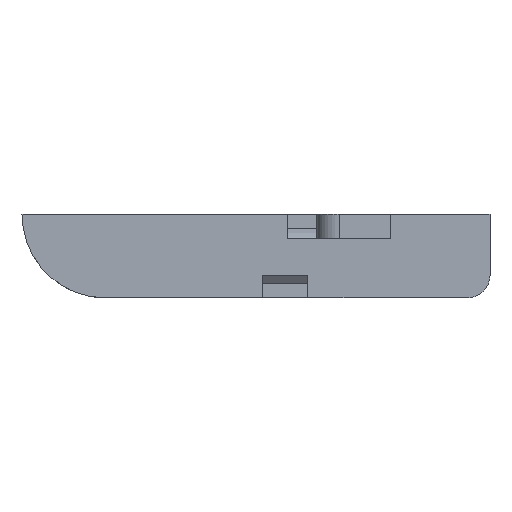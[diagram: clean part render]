
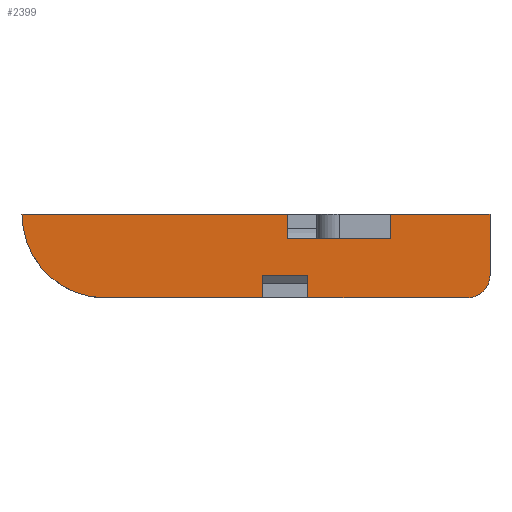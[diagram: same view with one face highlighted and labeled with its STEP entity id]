
A CAD part, left-side view. The second image highlights one B-rep face of the part: STEP entity #2399.
In plain terms, the highlighted planar face has unit normal (-1, 0, 0).
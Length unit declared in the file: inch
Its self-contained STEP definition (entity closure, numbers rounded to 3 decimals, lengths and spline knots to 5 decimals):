
#3 = DIRECTION ( 'NONE',  ( 0., 0., 1. ) ) ;
#45 = CIRCLE ( 'NONE', #3662, 0.19685 ) ;
#82 = DIRECTION ( 'NONE',  ( 0., 0., 1. ) ) ;
#101 = VERTEX_POINT ( 'NONE', #2831 ) ;
#126 = CARTESIAN_POINT ( 'NONE',  ( -5.00064, -0.47716, -0.73097 ) ) ;
#169 = EDGE_CURVE ( 'NONE', #2814, #2207, #1331, .T. ) ;
#211 = ORIENTED_EDGE ( 'NONE', *, *, #169, .T. ) ;
#276 = ORIENTED_EDGE ( 'NONE', *, *, #2015, .F. ) ;
#291 = DIRECTION ( 'NONE',  ( 0., -1., 0. ) ) ;
#300 = VECTOR ( 'NONE', #3422, 39.37008 ) ;
#414 = VERTEX_POINT ( 'NONE', #3549 ) ;
#424 = PLANE ( 'NONE',  #3716 ) ;
#447 = LINE ( 'NONE', #1786, #3554 ) ;
#448 = EDGE_CURVE ( 'NONE', #2156, #1865, #2391, .T. ) ;
#484 = CARTESIAN_POINT ( 'NONE',  ( -5.00064, -0.77841, -0.73097 ) ) ;
#490 = ORIENTED_EDGE ( 'NONE', *, *, #2410, .F. ) ;
#524 = CARTESIAN_POINT ( 'NONE',  ( -5.00064, -0.99151, -0.21654 ) ) ;
#542 = VERTEX_POINT ( 'NONE', #1649 ) ;
#549 = DIRECTION ( 'NONE',  ( 1., 0., 0. ) ) ;
#623 = VERTEX_POINT ( 'NONE', #524 ) ;
#681 = VECTOR ( 'NONE', #2763, 39.37008 ) ;
#728 = CARTESIAN_POINT ( 'NONE',  ( -5.00064, -1.17211, -0.53412 ) ) ;
#747 = ORIENTED_EDGE ( 'NONE', *, *, #1595, .T. ) ;
#834 = EDGE_CURVE ( 'NONE', #2156, #2940, #2741, .T. ) ;
#837 = LINE ( 'NONE', #2347, #3926 ) ;
#939 = CARTESIAN_POINT ( 'NONE',  ( -5.00064, -2.76317, -0.73097 ) ) ;
#994 = EDGE_CURVE ( 'NONE', #623, #3830, #837, .T. ) ;
#1031 = DIRECTION ( 'NONE',  ( -1., 0., 0. ) ) ;
#1116 = EDGE_CURVE ( 'NONE', #2940, #3830, #3651, .T. ) ;
#1156 = ORIENTED_EDGE ( 'NONE', *, *, #1116, .F. ) ;
#1210 = ORIENTED_EDGE ( 'NONE', *, *, #448, .T. ) ;
#1221 = EDGE_CURVE ( 'NONE', #623, #2922, #2472, .T. ) ;
#1230 = VERTEX_POINT ( 'NONE', #728 ) ;
#1263 = CARTESIAN_POINT ( 'NONE',  ( -5.00064, -2.56632, -0.73097 ) ) ;
#1272 = VECTOR ( 'NONE', #3, 39.37008 ) ;
#1275 = VECTOR ( 'NONE', #291, 39.37008 ) ;
#1288 = CARTESIAN_POINT ( 'NONE',  ( -5.00064, 2.30886, 0. ) ) ;
#1317 = CARTESIAN_POINT ( 'NONE',  ( -5.00064, -1.89702, 0. ) ) ;
#1321 = DIRECTION ( 'NONE',  ( 0., -1., 0. ) ) ;
#1331 = LINE ( 'NONE', #126, #3617 ) ;
#1423 = EDGE_CURVE ( 'NONE', #2922, #3621, #3414, .T. ) ;
#1460 = CARTESIAN_POINT ( 'NONE',  ( -5.00064, -1.17211, -0.73097 ) ) ;
#1595 = EDGE_CURVE ( 'NONE', #414, #542, #2075, .T. ) ;
#1611 = CARTESIAN_POINT ( 'NONE',  ( -5.00064, 0., -0.21654 ) ) ;
#1649 = CARTESIAN_POINT ( 'NONE',  ( -5.00064, -2.76317, 0. ) ) ;
#1740 = DIRECTION ( 'NONE',  ( 0., 0., 1. ) ) ;
#1745 = DIRECTION ( 'NONE',  ( 0., 0., 1. ) ) ;
#1786 = CARTESIAN_POINT ( 'NONE',  ( -5.00064, -0.77841, -0.73097 ) ) ;
#1805 = EDGE_CURVE ( 'NONE', #2207, #414, #45, .T. ) ;
#1865 = VERTEX_POINT ( 'NONE', #484 ) ;
#1909 = DIRECTION ( 'NONE',  ( -1., 0., 0. ) ) ;
#2015 = EDGE_CURVE ( 'NONE', #2814, #1230, #2841, .T. ) ;
#2058 = VECTOR ( 'NONE', #1745, 39.37008 ) ;
#2075 = LINE ( 'NONE', #939, #1272 ) ;
#2087 = DIRECTION ( 'NONE',  ( 0., 0., -1. ) ) ;
#2156 = VERTEX_POINT ( 'NONE', #3936 ) ;
#2207 = VERTEX_POINT ( 'NONE', #1263 ) ;
#2209 = CARTESIAN_POINT ( 'NONE',  ( -5.00064, -0.47716, -0.73097 ) ) ;
#2254 = EDGE_CURVE ( 'NONE', #3621, #542, #3895, .T. ) ;
#2266 = CARTESIAN_POINT ( 'NONE',  ( -5.00064, -1.17211, -0.73097 ) ) ;
#2276 = DIRECTION ( 'NONE',  ( 0., -1., 0. ) ) ;
#2290 = VECTOR ( 'NONE', #1321, 39.37008 ) ;
#2299 = CARTESIAN_POINT ( 'NONE',  ( -5.00064, -0.99151, 0. ) ) ;
#2345 = CARTESIAN_POINT ( 'NONE',  ( -5.00064, 0.59382, 0. ) ) ;
#2347 = CARTESIAN_POINT ( 'NONE',  ( -5.00064, -0.99151, 0. ) ) ;
#2391 = LINE ( 'NONE', #2209, #2290 ) ;
#2399 = ADVANCED_FACE ( 'NONE', ( #2699 ), #424, .T. ) ;
#2410 = EDGE_CURVE ( 'NONE', #1230, #101, #3392, .T. ) ;
#2472 = LINE ( 'NONE', #1611, #3364 ) ;
#2510 = CARTESIAN_POINT ( 'NONE',  ( -5.00064, 2.30886, -16.99949 ) ) ;
#2593 = CARTESIAN_POINT ( 'NONE',  ( -5.00064, -1.89702, -0.21654 ) ) ;
#2613 = EDGE_CURVE ( 'NONE', #101, #1865, #447, .T. ) ;
#2637 = DIRECTION ( 'NONE',  ( 0., 0., 1. ) ) ;
#2699 = FACE_OUTER_BOUND ( 'NONE', #2827, .T. ) ;
#2741 = CIRCLE ( 'NONE', #2833, 0.7313 ) ;
#2763 = DIRECTION ( 'NONE',  ( 0., -1., 0. ) ) ;
#2814 = VERTEX_POINT ( 'NONE', #2266 ) ;
#2827 = EDGE_LOOP ( 'NONE', ( #1156, #2835, #1210, #3582, #490, #276, #211, #3588, #747, #3279, #3070, #3122, #3595 ) ) ;
#2831 = CARTESIAN_POINT ( 'NONE',  ( -5.00064, -0.77841, -0.53412 ) ) ;
#2833 = AXIS2_PLACEMENT_3D ( 'NONE', #2345, #549, #2637 ) ;
#2835 = ORIENTED_EDGE ( 'NONE', *, *, #834, .F. ) ;
#2841 = LINE ( 'NONE', #1460, #2058 ) ;
#2922 = VERTEX_POINT ( 'NONE', #2593 ) ;
#2940 = VERTEX_POINT ( 'NONE', #3810 ) ;
#3070 = ORIENTED_EDGE ( 'NONE', *, *, #1423, .F. ) ;
#3114 = CARTESIAN_POINT ( 'NONE',  ( -5.00064, -1.17211, -0.53412 ) ) ;
#3122 = ORIENTED_EDGE ( 'NONE', *, *, #1221, .F. ) ;
#3128 = DIRECTION ( 'NONE',  ( 0., 0., 1. ) ) ;
#3215 = DIRECTION ( 'NONE',  ( 0., 0., 1. ) ) ;
#3277 = CARTESIAN_POINT ( 'NONE',  ( -5.00064, 2.30886, 0. ) ) ;
#3279 = ORIENTED_EDGE ( 'NONE', *, *, #2254, .F. ) ;
#3319 = VECTOR ( 'NONE', #3215, 39.37008 ) ;
#3364 = VECTOR ( 'NONE', #3703, 39.37008 ) ;
#3392 = LINE ( 'NONE', #3114, #300 ) ;
#3414 = LINE ( 'NONE', #3818, #3319 ) ;
#3422 = DIRECTION ( 'NONE',  ( 0., 1., 0. ) ) ;
#3549 = CARTESIAN_POINT ( 'NONE',  ( -5.00064, -2.76317, -0.53412 ) ) ;
#3554 = VECTOR ( 'NONE', #2087, 39.37008 ) ;
#3582 = ORIENTED_EDGE ( 'NONE', *, *, #2613, .F. ) ;
#3588 = ORIENTED_EDGE ( 'NONE', *, *, #1805, .T. ) ;
#3595 = ORIENTED_EDGE ( 'NONE', *, *, #994, .T. ) ;
#3617 = VECTOR ( 'NONE', #2276, 39.37008 ) ;
#3621 = VERTEX_POINT ( 'NONE', #1317 ) ;
#3651 = LINE ( 'NONE', #3277, #1275 ) ;
#3662 = AXIS2_PLACEMENT_3D ( 'NONE', #3705, #1909, #82 ) ;
#3703 = DIRECTION ( 'NONE',  ( 0., -1., 0. ) ) ;
#3705 = CARTESIAN_POINT ( 'NONE',  ( -5.00064, -2.56632, -0.53412 ) ) ;
#3716 = AXIS2_PLACEMENT_3D ( 'NONE', #2510, #1031, #3128 ) ;
#3810 = CARTESIAN_POINT ( 'NONE',  ( -5.00064, 1.32512, 0. ) ) ;
#3818 = CARTESIAN_POINT ( 'NONE',  ( -5.00064, -1.89702, -0.21654 ) ) ;
#3830 = VERTEX_POINT ( 'NONE', #2299 ) ;
#3895 = LINE ( 'NONE', #1288, #681 ) ;
#3926 = VECTOR ( 'NONE', #1740, 39.37008 ) ;
#3936 = CARTESIAN_POINT ( 'NONE',  ( -5.00064, 0.6158, -0.73097 ) ) ;
